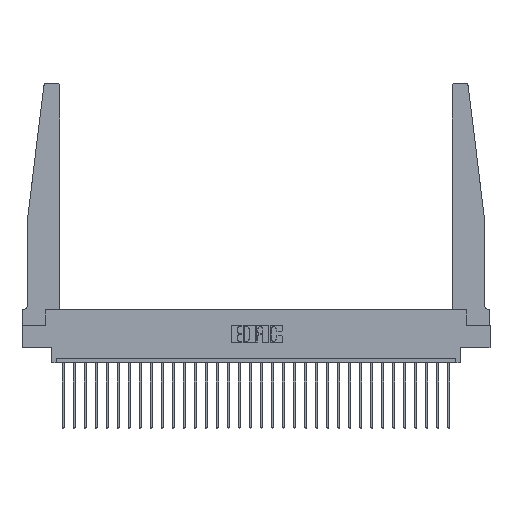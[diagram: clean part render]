
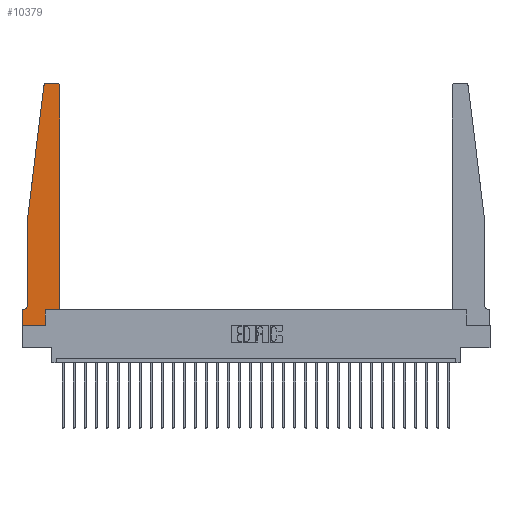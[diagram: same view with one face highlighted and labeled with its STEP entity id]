
A CAD part, top view. The second image highlights one B-rep face of the part: STEP entity #10379.
In plain terms, the highlighted planar face has unit normal (0, 0, 1).
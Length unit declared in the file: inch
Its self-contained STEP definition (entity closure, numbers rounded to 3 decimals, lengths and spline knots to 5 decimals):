
#30 = LINE ( 'NONE', #20149, #16619 ) ;
#159 = CARTESIAN_POINT ( 'NONE',  ( 0.425, 0.18, 0.37 ) ) ;
#1141 = DIRECTION ( 'NONE',  ( 0., -1., 0. ) ) ;
#1670 = CARTESIAN_POINT ( 'NONE',  ( 0., 0.1875, 0.37 ) ) ;
#1675 = VECTOR ( 'NONE', #8414, 39.37008 ) ;
#1778 = LINE ( 'NONE', #14428, #19708 ) ;
#2109 = LINE ( 'NONE', #18037, #15674 ) ;
#2220 = EDGE_CURVE ( 'NONE', #5969, #21069, #27481, .T. ) ;
#2442 = EDGE_CURVE ( 'NONE', #4525, #8317, #16912, .T. ) ;
#2448 = AXIS2_PLACEMENT_3D ( 'NONE', #11872, #24886, #18425 ) ;
#2484 = ORIENTED_EDGE ( 'NONE', *, *, #2442, .T. ) ;
#2856 = CARTESIAN_POINT ( 'NONE',  ( 0., 0.1875, 0.37 ) ) ;
#2898 = CIRCLE ( 'NONE', #2448, 0.05 ) ;
#2953 = EDGE_CURVE ( 'NONE', #13328, #4525, #30, .T. ) ;
#3205 = ORIENTED_EDGE ( 'NONE', *, *, #4174, .T. ) ;
#4174 = EDGE_CURVE ( 'NONE', #19414, #24988, #16535, .T. ) ;
#4362 = EDGE_CURVE ( 'NONE', #21069, #19414, #16853, .T. ) ;
#4459 = DIRECTION ( 'NONE',  ( 0., 0., 1. ) ) ;
#4525 = VERTEX_POINT ( 'NONE', #26743 ) ;
#4654 = PLANE ( 'NONE',  #16698 ) ;
#5072 = DIRECTION ( 'NONE',  ( -1., 0., 0. ) ) ;
#5969 = VERTEX_POINT ( 'NONE', #17419 ) ;
#6126 = EDGE_CURVE ( 'NONE', #15830, #22094, #2898, .T. ) ;
#6341 = ORIENTED_EDGE ( 'NONE', *, *, #2220, .T. ) ;
#6753 = ORIENTED_EDGE ( 'NONE', *, *, #2953, .T. ) ;
#6872 = VERTEX_POINT ( 'NONE', #18069 ) ;
#7612 = CARTESIAN_POINT ( 'NONE',  ( 0.065, 1.25, 0.37 ) ) ;
#7747 = DIRECTION ( 'NONE',  ( 1., 0., 0. ) ) ;
#7873 = EDGE_CURVE ( 'NONE', #22094, #13328, #2109, .T. ) ;
#7923 = CARTESIAN_POINT ( 'NONE',  ( 0.24675, 2.72367, 0.37 ) ) ;
#8010 = EDGE_CURVE ( 'NONE', #9545, #5969, #19351, .T. ) ;
#8317 = VERTEX_POINT ( 'NONE', #24044 ) ;
#8414 = DIRECTION ( 'NONE',  ( 0., 1., 0. ) ) ;
#9374 = ORIENTED_EDGE ( 'NONE', *, *, #4362, .T. ) ;
#9545 = VERTEX_POINT ( 'NONE', #22141 ) ;
#9738 = VECTOR ( 'NONE', #7747, 39.37008 ) ;
#10036 = CARTESIAN_POINT ( 'NONE',  ( 0.015, 0.1875, 0.37 ) ) ;
#10379 = ADVANCED_FACE ( 'NONE', ( #25237 ), #4654, .T. ) ;
#10519 = VECTOR ( 'NONE', #21887, 39.37008 ) ;
#10739 = CARTESIAN_POINT ( 'NONE',  ( 0.27653, 2.72, 0.37 ) ) ;
#11284 = DIRECTION ( 'NONE',  ( 0., 1., 0. ) ) ;
#11872 = CARTESIAN_POINT ( 'NONE',  ( 0.015, 0.2375, 0.37 ) ) ;
#12704 = ORIENTED_EDGE ( 'NONE', *, *, #6126, .T. ) ;
#13212 = CARTESIAN_POINT ( 'NONE',  ( 0.25, 2.75, 0.37 ) ) ;
#13328 = VERTEX_POINT ( 'NONE', #1670 ) ;
#13568 = DIRECTION ( 'NONE',  ( 1., 0., 0. ) ) ;
#14233 = AXIS2_PLACEMENT_3D ( 'NONE', #14783, #4459, #21388 ) ;
#14428 = CARTESIAN_POINT ( 'NONE',  ( 0.065, 1.25, 0.37 ) ) ;
#14783 = CARTESIAN_POINT ( 'NONE',  ( 0.395, 2.72, 0.37 ) ) ;
#15421 = CARTESIAN_POINT ( 'NONE',  ( 0.27653, 2.75, 0.37 ) ) ;
#15487 = DIRECTION ( 'NONE',  ( -1., 0., 0. ) ) ;
#15674 = VECTOR ( 'NONE', #5072, 39.37008 ) ;
#15830 = VERTEX_POINT ( 'NONE', #24575 ) ;
#16028 = VECTOR ( 'NONE', #11284, 39.37008 ) ;
#16232 = ORIENTED_EDGE ( 'NONE', *, *, #17113, .T. ) ;
#16535 = LINE ( 'NONE', #13212, #24678 ) ;
#16619 = VECTOR ( 'NONE', #22174, 39.37008 ) ;
#16698 = AXIS2_PLACEMENT_3D ( 'NONE', #2856, #19776, #13568 ) ;
#16853 = CIRCLE ( 'NONE', #14233, 0.03 ) ;
#16912 = LINE ( 'NONE', #20970, #9738 ) ;
#16939 = CARTESIAN_POINT ( 'NONE',  ( 0.425, 2.72, 0.37 ) ) ;
#17066 = EDGE_LOOP ( 'NONE', ( #3205, #22843, #21371, #16232, #12704, #27315, #6753, #2484, #26094, #21547, #6341, #9374 ) ) ;
#17113 = EDGE_CURVE ( 'NONE', #6872, #15830, #23259, .T. ) ;
#17290 = CARTESIAN_POINT ( 'NONE',  ( 0.395, 2.75, 0.37 ) ) ;
#17419 = CARTESIAN_POINT ( 'NONE',  ( 0.425, 0.18, 0.37 ) ) ;
#17639 = EDGE_CURVE ( 'NONE', #24988, #24669, #20157, .T. ) ;
#18037 = CARTESIAN_POINT ( 'NONE',  ( 0.065, 0.1875, 0.37 ) ) ;
#18069 = CARTESIAN_POINT ( 'NONE',  ( 0.065, 1.25, 0.37 ) ) ;
#18425 = DIRECTION ( 'NONE',  ( -1., 0., 0. ) ) ;
#18941 = EDGE_CURVE ( 'NONE', #24669, #6872, #1778, .T. ) ;
#19351 = LINE ( 'NONE', #26093, #10519 ) ;
#19414 = VERTEX_POINT ( 'NONE', #17290 ) ;
#19708 = VECTOR ( 'NONE', #22974, 39.37008 ) ;
#19776 = DIRECTION ( 'NONE',  ( 0., 0., 1. ) ) ;
#20149 = CARTESIAN_POINT ( 'NONE',  ( 0., 0., 0.37 ) ) ;
#20157 = CIRCLE ( 'NONE', #21134, 0.03 ) ;
#20751 = LINE ( 'NONE', #24055, #16028 ) ;
#20970 = CARTESIAN_POINT ( 'NONE',  ( 0., 0., 0.37 ) ) ;
#21069 = VERTEX_POINT ( 'NONE', #16939 ) ;
#21134 = AXIS2_PLACEMENT_3D ( 'NONE', #10739, #21297, #23602 ) ;
#21297 = DIRECTION ( 'NONE',  ( 0., 0., 1. ) ) ;
#21371 = ORIENTED_EDGE ( 'NONE', *, *, #18941, .T. ) ;
#21388 = DIRECTION ( 'NONE',  ( 1., 0., 0. ) ) ;
#21547 = ORIENTED_EDGE ( 'NONE', *, *, #8010, .T. ) ;
#21887 = DIRECTION ( 'NONE',  ( 1., 0., 0. ) ) ;
#22094 = VERTEX_POINT ( 'NONE', #10036 ) ;
#22141 = CARTESIAN_POINT ( 'NONE',  ( 0.2605, 0.18, 0.37 ) ) ;
#22174 = DIRECTION ( 'NONE',  ( 0., -1., 0. ) ) ;
#22547 = EDGE_CURVE ( 'NONE', #8317, #9545, #20751, .T. ) ;
#22843 = ORIENTED_EDGE ( 'NONE', *, *, #17639, .T. ) ;
#22974 = DIRECTION ( 'NONE',  ( -0.122, -0.992, 0. ) ) ;
#23259 = LINE ( 'NONE', #7612, #27333 ) ;
#23602 = DIRECTION ( 'NONE',  ( 1., 0., 0. ) ) ;
#24044 = CARTESIAN_POINT ( 'NONE',  ( 0.2605, 0., 0.37 ) ) ;
#24055 = CARTESIAN_POINT ( 'NONE',  ( 0.2605, 0.18, 0.37 ) ) ;
#24575 = CARTESIAN_POINT ( 'NONE',  ( 0.065, 0.2375, 0.37 ) ) ;
#24669 = VERTEX_POINT ( 'NONE', #7923 ) ;
#24678 = VECTOR ( 'NONE', #15487, 39.37008 ) ;
#24886 = DIRECTION ( 'NONE',  ( 0., 0., -1. ) ) ;
#24988 = VERTEX_POINT ( 'NONE', #15421 ) ;
#25237 = FACE_OUTER_BOUND ( 'NONE', #17066, .T. ) ;
#26093 = CARTESIAN_POINT ( 'NONE',  ( 0.425, 0.18, 0.37 ) ) ;
#26094 = ORIENTED_EDGE ( 'NONE', *, *, #22547, .T. ) ;
#26743 = CARTESIAN_POINT ( 'NONE',  ( 0., 0., 0.37 ) ) ;
#27315 = ORIENTED_EDGE ( 'NONE', *, *, #7873, .T. ) ;
#27333 = VECTOR ( 'NONE', #1141, 39.37008 ) ;
#27481 = LINE ( 'NONE', #159, #1675 ) ;
